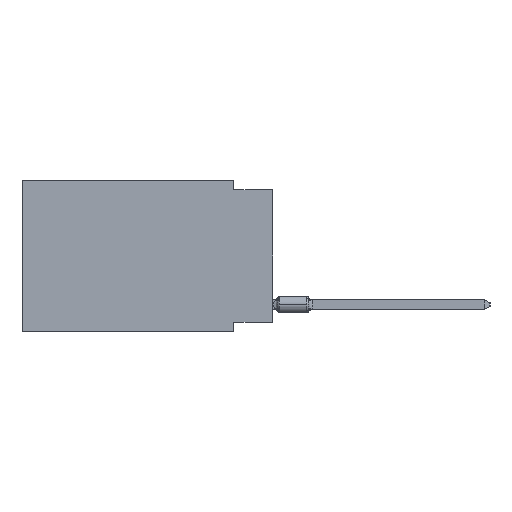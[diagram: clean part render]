
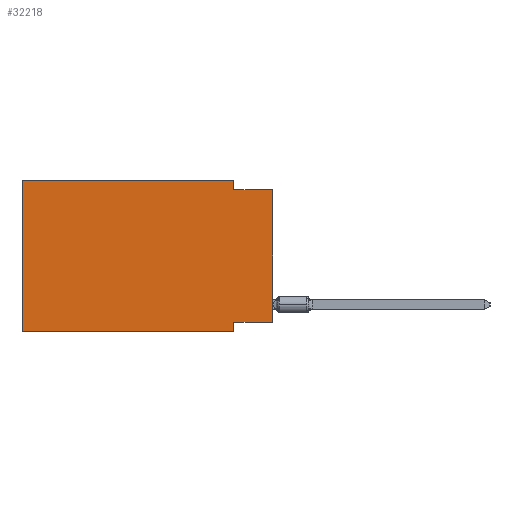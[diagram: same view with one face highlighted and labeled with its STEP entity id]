
A CAD part, left-side view. The second image highlights one B-rep face of the part: STEP entity #32218.
In plain terms, the highlighted planar face has unit normal (-1, 0, 0).
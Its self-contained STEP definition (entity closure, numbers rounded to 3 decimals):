
#512 = EDGE_CURVE ( 'NONE', #52392, #12600, #35025, .T. ) ;
#1248 = VERTEX_POINT ( 'NONE', #33541 ) ;
#2208 = CARTESIAN_POINT ( 'NONE',  ( 0., 2.54, -9.906 ) ) ;
#2725 = VERTEX_POINT ( 'NONE', #20302 ) ;
#4070 = LINE ( 'NONE', #46547, #29350 ) ;
#5731 = DIRECTION ( 'NONE',  ( 0., 0., 1. ) ) ;
#7299 = VECTOR ( 'NONE', #40186, 1000. ) ;
#9964 = CARTESIAN_POINT ( 'NONE',  ( 0., 16.383, 0. ) ) ;
#12600 = VERTEX_POINT ( 'NONE', #2208 ) ;
#12933 = VERTEX_POINT ( 'NONE', #22109 ) ;
#14284 = DIRECTION ( 'NONE',  ( 0., 0., -1. ) ) ;
#14577 = PLANE ( 'NONE',  #24474 ) ;
#14688 = LINE ( 'NONE', #42792, #35928 ) ;
#14860 = VECTOR ( 'NONE', #52982, 1000. ) ;
#15366 = ORIENTED_EDGE ( 'NONE', *, *, #20097, .F. ) ;
#15664 = VECTOR ( 'NONE', #26719, 1000. ) ;
#16094 = DIRECTION ( 'NONE',  ( 0., -1., 0. ) ) ;
#16210 = LINE ( 'NONE', #23588, #7299 ) ;
#16233 = EDGE_CURVE ( 'NONE', #2725, #52392, #50141, .T. ) ;
#16356 = EDGE_LOOP ( 'NONE', ( #20554, #33509, #15366, #30921, #25042, #23516, #42433, #19350 ) ) ;
#16894 = DIRECTION ( 'NONE',  ( 0., 0., -1. ) ) ;
#18152 = FACE_OUTER_BOUND ( 'NONE', #16356, .T. ) ;
#19350 = ORIENTED_EDGE ( 'NONE', *, *, #16233, .F. ) ;
#20097 = EDGE_CURVE ( 'NONE', #1248, #20677, #4070, .T. ) ;
#20302 = CARTESIAN_POINT ( 'NONE',  ( 0., 0., -9.271 ) ) ;
#20554 = ORIENTED_EDGE ( 'NONE', *, *, #35797, .T. ) ;
#20677 = VERTEX_POINT ( 'NONE', #46753 ) ;
#22109 = CARTESIAN_POINT ( 'NONE',  ( 0., 0., -0.635 ) ) ;
#23516 = ORIENTED_EDGE ( 'NONE', *, *, #34951, .T. ) ;
#23588 = CARTESIAN_POINT ( 'NONE',  ( 0., 16.383, -9.906 ) ) ;
#23947 = CARTESIAN_POINT ( 'NONE',  ( 0., 0., 0. ) ) ;
#24474 = AXIS2_PLACEMENT_3D ( 'NONE', #9964, #47266, #27417 ) ;
#24914 = EDGE_CURVE ( 'NONE', #31759, #1248, #40592, .T. ) ;
#25042 = ORIENTED_EDGE ( 'NONE', *, *, #48361, .F. ) ;
#25779 = EDGE_CURVE ( 'NONE', #20677, #12933, #48604, .T. ) ;
#26293 = VERTEX_POINT ( 'NONE', #36341 ) ;
#26719 = DIRECTION ( 'NONE',  ( 0., -1., 0. ) ) ;
#27417 = DIRECTION ( 'NONE',  ( 0., 0., -1. ) ) ;
#27942 = CARTESIAN_POINT ( 'NONE',  ( 0., 2.54, -9.271 ) ) ;
#29350 = VECTOR ( 'NONE', #16894, 1000. ) ;
#29491 = VECTOR ( 'NONE', #14284, 1000. ) ;
#30204 = CARTESIAN_POINT ( 'NONE',  ( 0., 16.383, 0. ) ) ;
#30921 = ORIENTED_EDGE ( 'NONE', *, *, #24914, .F. ) ;
#31759 = VERTEX_POINT ( 'NONE', #30204 ) ;
#32218 = ADVANCED_FACE ( 'NONE', ( #18152 ), #14577, .F. ) ;
#32375 = LINE ( 'NONE', #23947, #44879 ) ;
#33509 = ORIENTED_EDGE ( 'NONE', *, *, #25779, .F. ) ;
#33541 = CARTESIAN_POINT ( 'NONE',  ( 0., 2.54, 0. ) ) ;
#34951 = EDGE_CURVE ( 'NONE', #26293, #12600, #16210, .T. ) ;
#35025 = LINE ( 'NONE', #50771, #29491 ) ;
#35797 = EDGE_CURVE ( 'NONE', #2725, #12933, #32375, .T. ) ;
#35928 = VECTOR ( 'NONE', #5731, 1000. ) ;
#36341 = CARTESIAN_POINT ( 'NONE',  ( 0., 16.383, -9.906 ) ) ;
#38674 = CARTESIAN_POINT ( 'NONE',  ( 0., 0., -0.635 ) ) ;
#39940 = CARTESIAN_POINT ( 'NONE',  ( 0., 0., -9.271 ) ) ;
#40186 = DIRECTION ( 'NONE',  ( 0., -1., 0. ) ) ;
#40592 = LINE ( 'NONE', #53391, #45951 ) ;
#42433 = ORIENTED_EDGE ( 'NONE', *, *, #512, .F. ) ;
#42792 = CARTESIAN_POINT ( 'NONE',  ( 0., 16.383, 0. ) ) ;
#44879 = VECTOR ( 'NONE', #45129, 1000. ) ;
#45129 = DIRECTION ( 'NONE',  ( 0., 0., 1. ) ) ;
#45951 = VECTOR ( 'NONE', #16094, 1000. ) ;
#46547 = CARTESIAN_POINT ( 'NONE',  ( 0., 2.54, 0. ) ) ;
#46753 = CARTESIAN_POINT ( 'NONE',  ( 0., 2.54, -0.635 ) ) ;
#47266 = DIRECTION ( 'NONE',  ( 1., 0., 0. ) ) ;
#48361 = EDGE_CURVE ( 'NONE', #26293, #31759, #14688, .T. ) ;
#48604 = LINE ( 'NONE', #38674, #15664 ) ;
#50141 = LINE ( 'NONE', #39940, #14860 ) ;
#50771 = CARTESIAN_POINT ( 'NONE',  ( 0., 2.54, -9.906 ) ) ;
#52392 = VERTEX_POINT ( 'NONE', #27942 ) ;
#52982 = DIRECTION ( 'NONE',  ( 0., 1., 0. ) ) ;
#53391 = CARTESIAN_POINT ( 'NONE',  ( 0., 16.383, 0. ) ) ;
